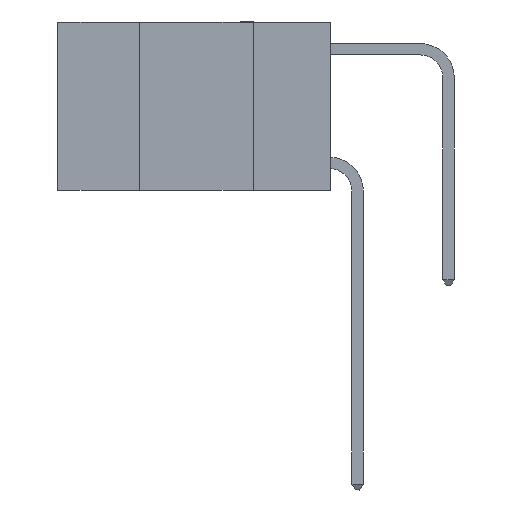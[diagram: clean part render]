
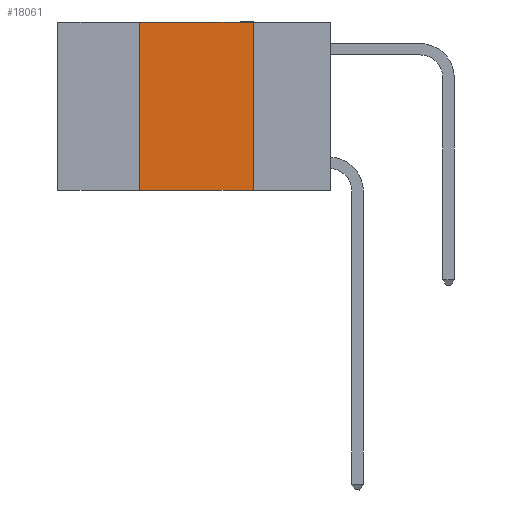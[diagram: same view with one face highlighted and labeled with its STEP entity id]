
A CAD part, left-side view. The second image highlights one B-rep face of the part: STEP entity #18061.
In plain terms, the highlighted planar face has unit normal (-1, 0, 0).
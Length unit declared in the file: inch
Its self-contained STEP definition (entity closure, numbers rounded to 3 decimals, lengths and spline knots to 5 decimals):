
#664 = CARTESIAN_POINT ( 'NONE',  ( 0., 0.6, 0. ) ) ;
#797 = AXIS2_PLACEMENT_3D ( 'NONE', #664, #13998, #5106 ) ;
#894 = VERTEX_POINT ( 'NONE', #2925 ) ;
#1584 = DIRECTION ( 'NONE',  ( 0., -1., 0. ) ) ;
#2925 = CARTESIAN_POINT ( 'NONE',  ( 0., 0.17, 0. ) ) ;
#2970 = CARTESIAN_POINT ( 'NONE',  ( 0., 0.6, 0. ) ) ;
#3108 = EDGE_CURVE ( 'NONE', #894, #16034, #15091, .T. ) ;
#3801 = DIRECTION ( 'NONE',  ( 0., 0., -1. ) ) ;
#3906 = LINE ( 'NONE', #2970, #11834 ) ;
#5106 = DIRECTION ( 'NONE',  ( 0., 0., -1. ) ) ;
#6169 = FACE_OUTER_BOUND ( 'NONE', #7241, .T. ) ;
#6237 = CARTESIAN_POINT ( 'NONE',  ( 0., 0.42, 0. ) ) ;
#7140 = ORIENTED_EDGE ( 'NONE', *, *, #13040, .F. ) ;
#7241 = EDGE_LOOP ( 'NONE', ( #8967, #18666, #7140, #9530 ) ) ;
#7300 = LINE ( 'NONE', #14227, #14713 ) ;
#7483 = EDGE_CURVE ( 'NONE', #8883, #894, #3906, .T. ) ;
#8169 = CARTESIAN_POINT ( 'NONE',  ( 0., 0.42, -0.37 ) ) ;
#8883 = VERTEX_POINT ( 'NONE', #6237 ) ;
#8967 = ORIENTED_EDGE ( 'NONE', *, *, #3108, .F. ) ;
#8975 = CARTESIAN_POINT ( 'NONE',  ( 0., 0.6, -0.37 ) ) ;
#9530 = ORIENTED_EDGE ( 'NONE', *, *, #9577, .T. ) ;
#9577 = EDGE_CURVE ( 'NONE', #15547, #16034, #17962, .T. ) ;
#10115 = VECTOR ( 'NONE', #1584, 39.37008 ) ;
#11170 = VECTOR ( 'NONE', #3801, 39.37008 ) ;
#11834 = VECTOR ( 'NONE', #11870, 39.37008 ) ;
#11870 = DIRECTION ( 'NONE',  ( 0., -1., 0. ) ) ;
#13040 = EDGE_CURVE ( 'NONE', #15547, #8883, #7300, .T. ) ;
#13625 = CARTESIAN_POINT ( 'NONE',  ( 0., 0.17, -0.37 ) ) ;
#13998 = DIRECTION ( 'NONE',  ( 1., 0., 0. ) ) ;
#14185 = CARTESIAN_POINT ( 'NONE',  ( 0., 0.17, 0. ) ) ;
#14227 = CARTESIAN_POINT ( 'NONE',  ( 0., 0.42, 0. ) ) ;
#14713 = VECTOR ( 'NONE', #15773, 39.37008 ) ;
#15091 = LINE ( 'NONE', #14185, #11170 ) ;
#15547 = VERTEX_POINT ( 'NONE', #8169 ) ;
#15773 = DIRECTION ( 'NONE',  ( 0., 0., 1. ) ) ;
#16034 = VERTEX_POINT ( 'NONE', #13625 ) ;
#16904 = PLANE ( 'NONE',  #797 ) ;
#17962 = LINE ( 'NONE', #8975, #10115 ) ;
#18061 = ADVANCED_FACE ( 'NONE', ( #6169 ), #16904, .F. ) ;
#18666 = ORIENTED_EDGE ( 'NONE', *, *, #7483, .F. ) ;
